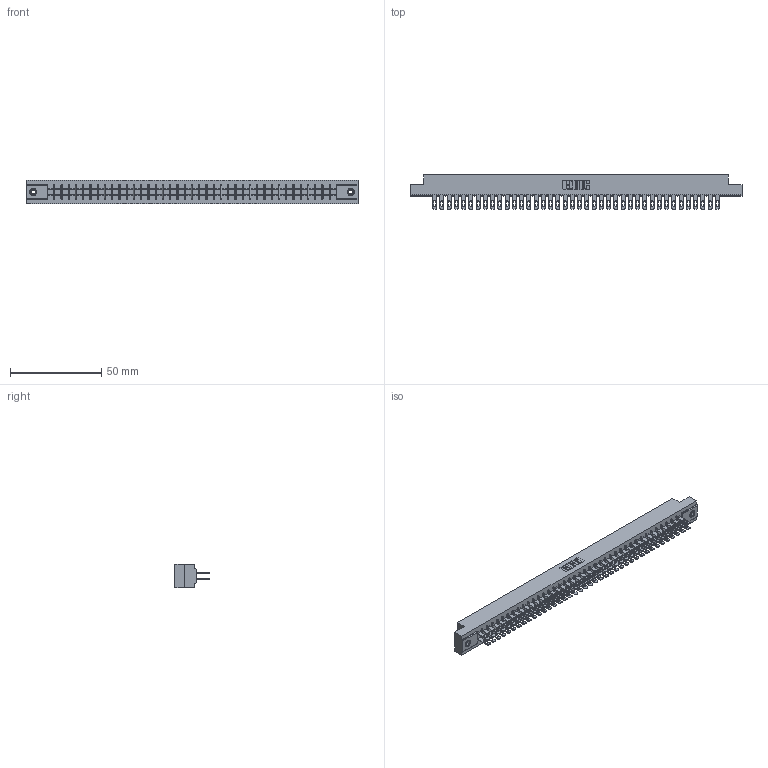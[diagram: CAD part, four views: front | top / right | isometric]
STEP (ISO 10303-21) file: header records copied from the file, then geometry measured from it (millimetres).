
FILE_DESCRIPTION (( 'STEP AP203' ), '1' );
FILE_NAME ('305-080-500-508.STEP', '2019-09-10T09:40:19', ( '' ), ( '' ), 'SwSTEP 2.0', 'SolidWorks 2016', '' );
FILE_SCHEMA (( 'CONFIG_CONTROL_DESIGN' ));
Length unit declared in the file: inch
Products named in the file (4): 305-290-001_500; 305-080-500-508; 305 Part_.156 Dia; 345-250-001_345-250-003-102
Assembly tree (83 placements, depth 2):
  305-080-500-508
    305 Part_.156 Dia
    305-290-001_500  x80
    345-250-001_345-250-003-102  x2
Bounding box: 181.51 x 18.85 x 12.7 mm (x, y, z)
Volume: 18611.4 mm3; surface area: 26104.8 mm2
Topology: 83 solids, 83 shells, 4176 faces, 11932 edges, 7732 vertices
Faces by surface type: plane 2340, cylinder 1660, sphere 160, cone 12, torus 4
Entity records: 44760 total; most frequent: CARTESIAN_POINT 7389, ORIENTED_EDGE 7328, DIRECTION 7162, EDGE_CURVE 3664, VECTOR 2956, LINE 2956, VERTEX_POINT 2330, AXIS2_PLACEMENT_3D 2103
